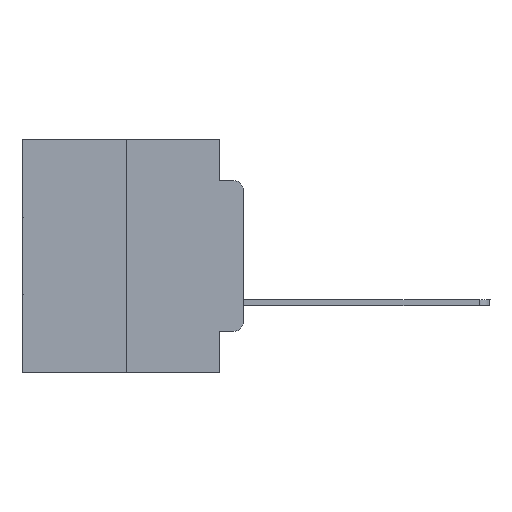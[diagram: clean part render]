
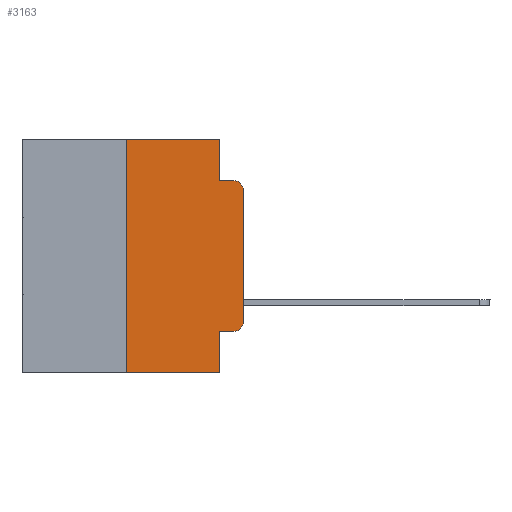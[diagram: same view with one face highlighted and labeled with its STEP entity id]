
A CAD part, left-side view. The second image highlights one B-rep face of the part: STEP entity #3163.
In plain terms, the highlighted planar face has unit normal (-1, 0, 0).
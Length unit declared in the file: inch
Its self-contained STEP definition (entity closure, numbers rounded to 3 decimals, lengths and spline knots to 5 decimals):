
#287 = CARTESIAN_POINT ( 'NONE',  ( 0., 0.473, -0.5 ) ) ;
#364 = AXIS2_PLACEMENT_3D ( 'NONE', #9549, #24992, #7128 ) ;
#481 = EDGE_CURVE ( 'NONE', #10866, #9420, #18596, .T. ) ;
#523 = DIRECTION ( 'NONE',  ( 0., 0., -1. ) ) ;
#745 = EDGE_LOOP ( 'NONE', ( #28494, #2661, #10074, #2584, #26523, #27898, #22546, #22440, #8019, #25806 ) ) ;
#1743 = VECTOR ( 'NONE', #12986, 39.37008 ) ;
#2165 = CARTESIAN_POINT ( 'NONE',  ( 0., 0.25, 0. ) ) ;
#2411 = VECTOR ( 'NONE', #6693, 39.37008 ) ;
#2530 = DIRECTION ( 'NONE',  ( -1., 0., 0. ) ) ;
#2584 = ORIENTED_EDGE ( 'NONE', *, *, #12413, .F. ) ;
#2661 = ORIENTED_EDGE ( 'NONE', *, *, #481, .T. ) ;
#2740 = CARTESIAN_POINT ( 'NONE',  ( 0., 0.02, -0.4115 ) ) ;
#3163 = ADVANCED_FACE ( 'NONE', ( #9561 ), #12076, .F. ) ;
#4023 = CARTESIAN_POINT ( 'NONE',  ( 0., 0.02, -0.1085 ) ) ;
#4577 = VECTOR ( 'NONE', #23663, 39.37008 ) ;
#4809 = DIRECTION ( 'NONE',  ( 0., 0., -1. ) ) ;
#4873 = VECTOR ( 'NONE', #20129, 39.37008 ) ;
#6515 = VERTEX_POINT ( 'NONE', #2165 ) ;
#6590 = AXIS2_PLACEMENT_3D ( 'NONE', #13807, #22519, #4809 ) ;
#6649 = CIRCLE ( 'NONE', #364, 0.02 ) ;
#6693 = DIRECTION ( 'NONE',  ( 0., -1., 0. ) ) ;
#6970 = CARTESIAN_POINT ( 'NONE',  ( 0., 0.051, 0. ) ) ;
#7128 = DIRECTION ( 'NONE',  ( 0., 0., -1. ) ) ;
#7823 = DIRECTION ( 'NONE',  ( 0., 0., 1. ) ) ;
#8018 = VERTEX_POINT ( 'NONE', #19682 ) ;
#8019 = ORIENTED_EDGE ( 'NONE', *, *, #23519, .T. ) ;
#8302 = LINE ( 'NONE', #19850, #2411 ) ;
#8477 = CARTESIAN_POINT ( 'NONE',  ( 0., 0., -0.1085 ) ) ;
#8951 = EDGE_CURVE ( 'NONE', #17278, #16935, #24431, .T. ) ;
#9420 = VERTEX_POINT ( 'NONE', #13152 ) ;
#9549 = CARTESIAN_POINT ( 'NONE',  ( 0., 0.02, -0.3915 ) ) ;
#9561 = FACE_OUTER_BOUND ( 'NONE', #745, .T. ) ;
#10074 = ORIENTED_EDGE ( 'NONE', *, *, #23723, .F. ) ;
#10456 = LINE ( 'NONE', #26093, #4577 ) ;
#10866 = VERTEX_POINT ( 'NONE', #8477 ) ;
#11153 = VERTEX_POINT ( 'NONE', #15871 ) ;
#12076 = PLANE ( 'NONE',  #6590 ) ;
#12345 = EDGE_CURVE ( 'NONE', #6515, #27035, #24603, .T. ) ;
#12413 = EDGE_CURVE ( 'NONE', #27035, #8018, #12865, .T. ) ;
#12592 = EDGE_CURVE ( 'NONE', #14223, #6515, #10456, .T. ) ;
#12637 = VECTOR ( 'NONE', #18033, 39.37008 ) ;
#12865 = LINE ( 'NONE', #28248, #25305 ) ;
#12887 = CARTESIAN_POINT ( 'NONE',  ( 0., 0.051, -0.4115 ) ) ;
#12986 = DIRECTION ( 'NONE',  ( 0., -1., 0. ) ) ;
#13152 = CARTESIAN_POINT ( 'NONE',  ( 0., 0.02, -0.0885 ) ) ;
#13807 = CARTESIAN_POINT ( 'NONE',  ( 0., 0.473, 0. ) ) ;
#14223 = VERTEX_POINT ( 'NONE', #25558 ) ;
#14396 = VECTOR ( 'NONE', #24126, 39.37008 ) ;
#14720 = CARTESIAN_POINT ( 'NONE',  ( 0., 0.473, 0. ) ) ;
#15036 = CARTESIAN_POINT ( 'NONE',  ( 0., 0.051, 0. ) ) ;
#15871 = CARTESIAN_POINT ( 'NONE',  ( 0., 0., -0.3915 ) ) ;
#16012 = CARTESIAN_POINT ( 'NONE',  ( 0., 0.051, -0.5 ) ) ;
#16846 = CARTESIAN_POINT ( 'NONE',  ( 0., 0.051, -0.4115 ) ) ;
#16935 = VERTEX_POINT ( 'NONE', #16012 ) ;
#17278 = VERTEX_POINT ( 'NONE', #16846 ) ;
#17603 = VERTEX_POINT ( 'NONE', #2740 ) ;
#18033 = DIRECTION ( 'NONE',  ( 0., -1., 0. ) ) ;
#18596 = CIRCLE ( 'NONE', #25245, 0.02 ) ;
#18866 = EDGE_CURVE ( 'NONE', #11153, #10866, #26507, .T. ) ;
#19682 = CARTESIAN_POINT ( 'NONE',  ( 0., 0.051, -0.0885 ) ) ;
#19850 = CARTESIAN_POINT ( 'NONE',  ( 0., 0.051, -0.0885 ) ) ;
#20129 = DIRECTION ( 'NONE',  ( 0., -1., 0. ) ) ;
#20672 = CARTESIAN_POINT ( 'NONE',  ( 0., 0., 0. ) ) ;
#22440 = ORIENTED_EDGE ( 'NONE', *, *, #8951, .F. ) ;
#22519 = DIRECTION ( 'NONE',  ( 1., 0., 0. ) ) ;
#22546 = ORIENTED_EDGE ( 'NONE', *, *, #25694, .T. ) ;
#22808 = LINE ( 'NONE', #12887, #1743 ) ;
#23519 = EDGE_CURVE ( 'NONE', #17278, #17603, #22808, .T. ) ;
#23663 = DIRECTION ( 'NONE',  ( 0., 0., 1. ) ) ;
#23723 = EDGE_CURVE ( 'NONE', #8018, #9420, #8302, .T. ) ;
#24126 = DIRECTION ( 'NONE',  ( 0., 0., -1. ) ) ;
#24431 = LINE ( 'NONE', #15036, #14396 ) ;
#24603 = LINE ( 'NONE', #14720, #4873 ) ;
#24992 = DIRECTION ( 'NONE',  ( -1., 0., 0. ) ) ;
#25084 = LINE ( 'NONE', #287, #12637 ) ;
#25245 = AXIS2_PLACEMENT_3D ( 'NONE', #4023, #2530, #523 ) ;
#25305 = VECTOR ( 'NONE', #26296, 39.37008 ) ;
#25558 = CARTESIAN_POINT ( 'NONE',  ( 0., 0.25, -0.5 ) ) ;
#25694 = EDGE_CURVE ( 'NONE', #14223, #16935, #25084, .T. ) ;
#25806 = ORIENTED_EDGE ( 'NONE', *, *, #27552, .T. ) ;
#26093 = CARTESIAN_POINT ( 'NONE',  ( 0., 0.25, 0. ) ) ;
#26296 = DIRECTION ( 'NONE',  ( 0., 0., -1. ) ) ;
#26507 = LINE ( 'NONE', #20672, #27884 ) ;
#26523 = ORIENTED_EDGE ( 'NONE', *, *, #12345, .F. ) ;
#27035 = VERTEX_POINT ( 'NONE', #6970 ) ;
#27552 = EDGE_CURVE ( 'NONE', #17603, #11153, #6649, .T. ) ;
#27884 = VECTOR ( 'NONE', #7823, 39.37008 ) ;
#27898 = ORIENTED_EDGE ( 'NONE', *, *, #12592, .F. ) ;
#28248 = CARTESIAN_POINT ( 'NONE',  ( 0., 0.051, 0. ) ) ;
#28494 = ORIENTED_EDGE ( 'NONE', *, *, #18866, .T. ) ;
